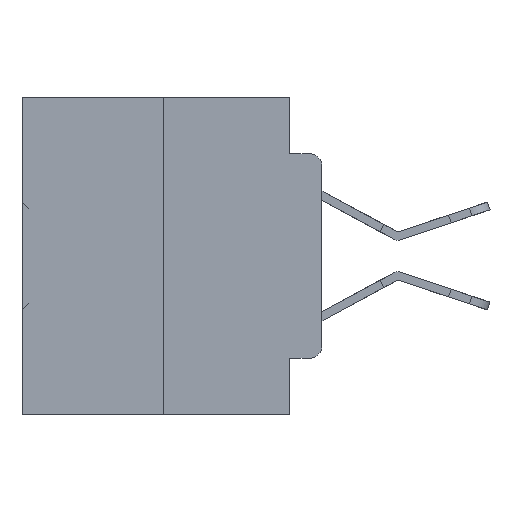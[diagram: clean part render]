
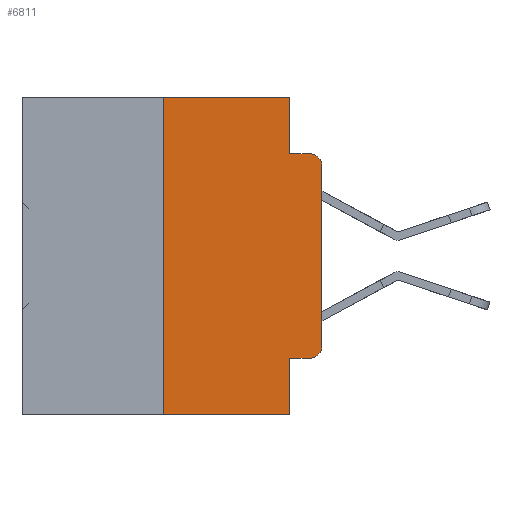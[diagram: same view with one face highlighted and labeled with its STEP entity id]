
A CAD part, left-side view. The second image highlights one B-rep face of the part: STEP entity #6811.
In plain terms, the highlighted planar face has unit normal (-1, 0, 0).
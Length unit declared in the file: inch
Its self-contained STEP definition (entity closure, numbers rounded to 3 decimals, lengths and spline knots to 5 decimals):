
#230 = EDGE_CURVE ( 'NONE', #6608, #13144, #37058, .T. ) ;
#584 = CARTESIAN_POINT ( 'NONE',  ( 0., 0.051, -0.4115 ) ) ;
#716 = EDGE_CURVE ( 'NONE', #7228, #22689, #4986, .T. ) ;
#1813 = DIRECTION ( 'NONE',  ( 0., -1., 0. ) ) ;
#1881 = VECTOR ( 'NONE', #12661, 39.37008 ) ;
#2111 = CARTESIAN_POINT ( 'NONE',  ( 0., 0.051, -0.0885 ) ) ;
#3050 = ORIENTED_EDGE ( 'NONE', *, *, #13520, .T. ) ;
#3149 = ORIENTED_EDGE ( 'NONE', *, *, #13997, .T. ) ;
#3514 = EDGE_CURVE ( 'NONE', #27295, #6608, #21715, .T. ) ;
#3754 = VECTOR ( 'NONE', #20341, 39.37008 ) ;
#3884 = CIRCLE ( 'NONE', #29315, 0.02 ) ;
#4515 = VECTOR ( 'NONE', #25003, 39.37008 ) ;
#4986 = LINE ( 'NONE', #31604, #3754 ) ;
#6347 = ORIENTED_EDGE ( 'NONE', *, *, #230, .F. ) ;
#6608 = VERTEX_POINT ( 'NONE', #13701 ) ;
#6619 = CARTESIAN_POINT ( 'NONE',  ( 0., 0.473, 0. ) ) ;
#6652 = CARTESIAN_POINT ( 'NONE',  ( 0., 0., 0. ) ) ;
#6811 = ADVANCED_FACE ( 'NONE', ( #14991 ), #26847, .F. ) ;
#6924 = LINE ( 'NONE', #22281, #20372 ) ;
#6957 = ORIENTED_EDGE ( 'NONE', *, *, #16270, .T. ) ;
#7228 = VERTEX_POINT ( 'NONE', #584 ) ;
#7355 = VERTEX_POINT ( 'NONE', #37025 ) ;
#8528 = CIRCLE ( 'NONE', #17836, 0.02 ) ;
#9978 = VECTOR ( 'NONE', #15654, 39.37008 ) ;
#10103 = DIRECTION ( 'NONE',  ( 0., 0., -1. ) ) ;
#10224 = EDGE_LOOP ( 'NONE', ( #28668, #3149, #21846, #6347, #27523, #25502, #11724, #36619, #3050, #6957 ) ) ;
#10225 = DIRECTION ( 'NONE',  ( 0., 0., 1. ) ) ;
#10932 = LINE ( 'NONE', #16570, #38088 ) ;
#11147 = DIRECTION ( 'NONE',  ( 0., 0., -1. ) ) ;
#11724 = ORIENTED_EDGE ( 'NONE', *, *, #25001, .T. ) ;
#12633 = DIRECTION ( 'NONE',  ( 0., 0., -1. ) ) ;
#12661 = DIRECTION ( 'NONE',  ( 0., 0., 1. ) ) ;
#13144 = VERTEX_POINT ( 'NONE', #34715 ) ;
#13151 = CARTESIAN_POINT ( 'NONE',  ( 0., 0.473, 0. ) ) ;
#13520 = EDGE_CURVE ( 'NONE', #7228, #31500, #21481, .T. ) ;
#13701 = CARTESIAN_POINT ( 'NONE',  ( 0., 0.051, 0. ) ) ;
#13952 = LINE ( 'NONE', #2111, #36993 ) ;
#13997 = EDGE_CURVE ( 'NONE', #7355, #16928, #3884, .T. ) ;
#14991 = FACE_OUTER_BOUND ( 'NONE', #10224, .T. ) ;
#15398 = VECTOR ( 'NONE', #34168, 39.37008 ) ;
#15515 = CARTESIAN_POINT ( 'NONE',  ( 0., 0.051, -0.5 ) ) ;
#15654 = DIRECTION ( 'NONE',  ( 0., -1., 0. ) ) ;
#15712 = EDGE_CURVE ( 'NONE', #13144, #16928, #13952, .T. ) ;
#15751 = DIRECTION ( 'NONE',  ( -1., 0., 0. ) ) ;
#16270 = EDGE_CURVE ( 'NONE', #31500, #27677, #8528, .T. ) ;
#16392 = CARTESIAN_POINT ( 'NONE',  ( 0., 0.02, -0.3915 ) ) ;
#16570 = CARTESIAN_POINT ( 'NONE',  ( 0., 0.473, -0.5 ) ) ;
#16928 = VERTEX_POINT ( 'NONE', #18214 ) ;
#17091 = EDGE_CURVE ( 'NONE', #30921, #27295, #6924, .T. ) ;
#17836 = AXIS2_PLACEMENT_3D ( 'NONE', #16392, #19474, #11147 ) ;
#18214 = CARTESIAN_POINT ( 'NONE',  ( 0., 0.02, -0.0885 ) ) ;
#18483 = DIRECTION ( 'NONE',  ( 1., 0., 0. ) ) ;
#19342 = EDGE_CURVE ( 'NONE', #27677, #7355, #27622, .T. ) ;
#19360 = CARTESIAN_POINT ( 'NONE',  ( 0., 0.02, -0.4115 ) ) ;
#19474 = DIRECTION ( 'NONE',  ( -1., 0., 0. ) ) ;
#20341 = DIRECTION ( 'NONE',  ( 0., 0., -1. ) ) ;
#20372 = VECTOR ( 'NONE', #10225, 39.37008 ) ;
#20820 = AXIS2_PLACEMENT_3D ( 'NONE', #6619, #18483, #12633 ) ;
#21481 = LINE ( 'NONE', #33323, #9978 ) ;
#21581 = CARTESIAN_POINT ( 'NONE',  ( 0., 0.25, -0.5 ) ) ;
#21715 = LINE ( 'NONE', #13151, #4515 ) ;
#21846 = ORIENTED_EDGE ( 'NONE', *, *, #15712, .F. ) ;
#22281 = CARTESIAN_POINT ( 'NONE',  ( 0., 0.25, 0. ) ) ;
#22340 = CARTESIAN_POINT ( 'NONE',  ( 0., 0.051, 0. ) ) ;
#22689 = VERTEX_POINT ( 'NONE', #15515 ) ;
#22693 = DIRECTION ( 'NONE',  ( 0., -1., 0. ) ) ;
#25001 = EDGE_CURVE ( 'NONE', #30921, #22689, #10932, .T. ) ;
#25003 = DIRECTION ( 'NONE',  ( 0., -1., 0. ) ) ;
#25502 = ORIENTED_EDGE ( 'NONE', *, *, #17091, .F. ) ;
#26198 = CARTESIAN_POINT ( 'NONE',  ( 0., 0.25, 0. ) ) ;
#26847 = PLANE ( 'NONE',  #20820 ) ;
#27295 = VERTEX_POINT ( 'NONE', #26198 ) ;
#27324 = CARTESIAN_POINT ( 'NONE',  ( 0., 0., -0.3915 ) ) ;
#27523 = ORIENTED_EDGE ( 'NONE', *, *, #3514, .F. ) ;
#27622 = LINE ( 'NONE', #6652, #1881 ) ;
#27677 = VERTEX_POINT ( 'NONE', #27324 ) ;
#28668 = ORIENTED_EDGE ( 'NONE', *, *, #19342, .T. ) ;
#29315 = AXIS2_PLACEMENT_3D ( 'NONE', #36869, #15751, #10103 ) ;
#30921 = VERTEX_POINT ( 'NONE', #21581 ) ;
#31500 = VERTEX_POINT ( 'NONE', #19360 ) ;
#31604 = CARTESIAN_POINT ( 'NONE',  ( 0., 0.051, 0. ) ) ;
#33323 = CARTESIAN_POINT ( 'NONE',  ( 0., 0.051, -0.4115 ) ) ;
#34168 = DIRECTION ( 'NONE',  ( 0., 0., -1. ) ) ;
#34715 = CARTESIAN_POINT ( 'NONE',  ( 0., 0.051, -0.0885 ) ) ;
#36619 = ORIENTED_EDGE ( 'NONE', *, *, #716, .F. ) ;
#36869 = CARTESIAN_POINT ( 'NONE',  ( 0., 0.02, -0.1085 ) ) ;
#36993 = VECTOR ( 'NONE', #22693, 39.37008 ) ;
#37025 = CARTESIAN_POINT ( 'NONE',  ( 0., 0., -0.1085 ) ) ;
#37058 = LINE ( 'NONE', #22340, #15398 ) ;
#38088 = VECTOR ( 'NONE', #1813, 39.37008 ) ;
